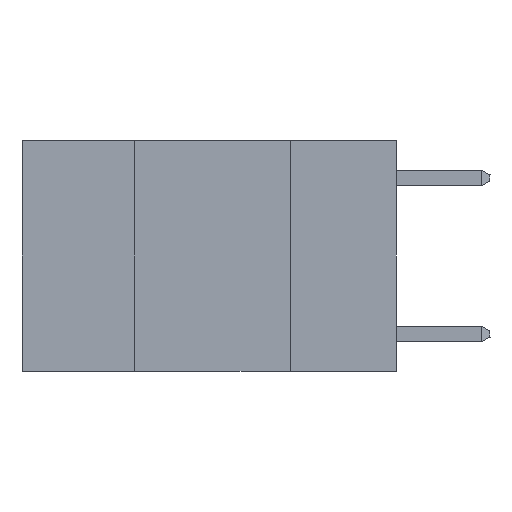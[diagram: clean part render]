
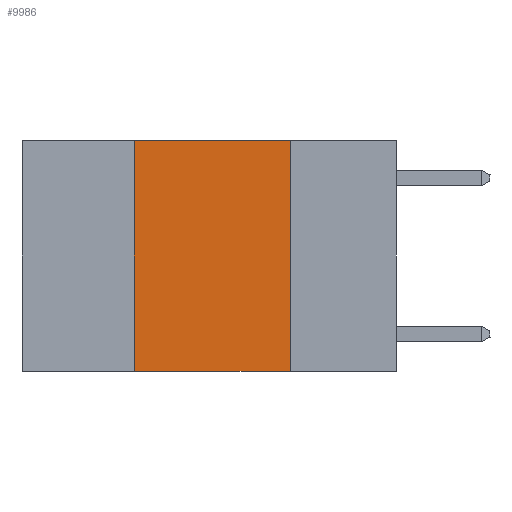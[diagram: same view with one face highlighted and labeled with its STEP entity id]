
A CAD part, left-side view. The second image highlights one B-rep face of the part: STEP entity #9986.
In plain terms, the highlighted planar face has unit normal (-1, 0, 0).
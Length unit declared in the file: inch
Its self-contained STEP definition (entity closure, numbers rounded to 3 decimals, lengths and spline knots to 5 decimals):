
#56 = VECTOR ( 'NONE', #11271, 39.37008 ) ;
#139 = CARTESIAN_POINT ( 'NONE',  ( 0., 0.6, -0.37 ) ) ;
#500 = CARTESIAN_POINT ( 'NONE',  ( 0., 0.17, 0. ) ) ;
#532 = DIRECTION ( 'NONE',  ( 0., 0., -1. ) ) ;
#719 = LINE ( 'NONE', #11097, #56 ) ;
#920 = EDGE_CURVE ( 'NONE', #4338, #11294, #3972, .T. ) ;
#1440 = FACE_OUTER_BOUND ( 'NONE', #10083, .T. ) ;
#1723 = EDGE_CURVE ( 'NONE', #4338, #4522, #5429, .T. ) ;
#3061 = PLANE ( 'NONE',  #8041 ) ;
#3318 = VERTEX_POINT ( 'NONE', #500 ) ;
#3641 = ORIENTED_EDGE ( 'NONE', *, *, #1723, .T. ) ;
#3880 = EDGE_CURVE ( 'NONE', #11294, #3318, #719, .T. ) ;
#3972 = LINE ( 'NONE', #7385, #7071 ) ;
#4102 = LINE ( 'NONE', #8637, #6808 ) ;
#4207 = DIRECTION ( 'NONE',  ( 0., 0., -1. ) ) ;
#4338 = VERTEX_POINT ( 'NONE', #9756 ) ;
#4522 = VERTEX_POINT ( 'NONE', #11227 ) ;
#4930 = CARTESIAN_POINT ( 'NONE',  ( 0., 0.6, 0. ) ) ;
#5427 = ORIENTED_EDGE ( 'NONE', *, *, #3880, .F. ) ;
#5429 = LINE ( 'NONE', #139, #10055 ) ;
#6808 = VECTOR ( 'NONE', #4207, 39.37008 ) ;
#7071 = VECTOR ( 'NONE', #9195, 39.37008 ) ;
#7385 = CARTESIAN_POINT ( 'NONE',  ( 0., 0.42, 0. ) ) ;
#7421 = ORIENTED_EDGE ( 'NONE', *, *, #7926, .F. ) ;
#7926 = EDGE_CURVE ( 'NONE', #3318, #4522, #4102, .T. ) ;
#8041 = AXIS2_PLACEMENT_3D ( 'NONE', #4930, #11033, #532 ) ;
#8120 = ORIENTED_EDGE ( 'NONE', *, *, #920, .F. ) ;
#8637 = CARTESIAN_POINT ( 'NONE',  ( 0., 0.17, 0. ) ) ;
#9195 = DIRECTION ( 'NONE',  ( 0., 0., 1. ) ) ;
#9434 = CARTESIAN_POINT ( 'NONE',  ( 0., 0.42, 0. ) ) ;
#9756 = CARTESIAN_POINT ( 'NONE',  ( 0., 0.42, -0.37 ) ) ;
#9986 = ADVANCED_FACE ( 'NONE', ( #1440 ), #3061, .F. ) ;
#10055 = VECTOR ( 'NONE', #10620, 39.37008 ) ;
#10083 = EDGE_LOOP ( 'NONE', ( #7421, #5427, #8120, #3641 ) ) ;
#10620 = DIRECTION ( 'NONE',  ( 0., -1., 0. ) ) ;
#11033 = DIRECTION ( 'NONE',  ( 1., 0., 0. ) ) ;
#11097 = CARTESIAN_POINT ( 'NONE',  ( 0., 0.6, 0. ) ) ;
#11227 = CARTESIAN_POINT ( 'NONE',  ( 0., 0.17, -0.37 ) ) ;
#11271 = DIRECTION ( 'NONE',  ( 0., -1., 0. ) ) ;
#11294 = VERTEX_POINT ( 'NONE', #9434 ) ;
